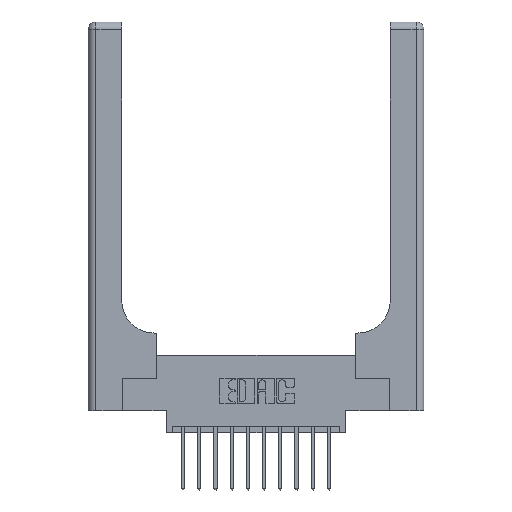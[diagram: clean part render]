
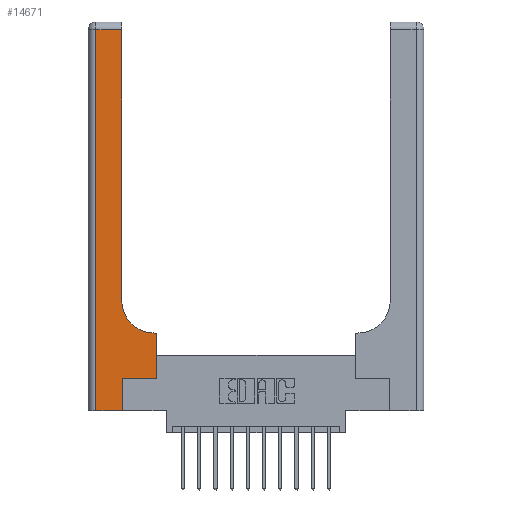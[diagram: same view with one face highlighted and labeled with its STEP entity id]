
A CAD part, top view. The second image highlights one B-rep face of the part: STEP entity #14671.
In plain terms, the highlighted planar face has unit normal (0, 0, 1).
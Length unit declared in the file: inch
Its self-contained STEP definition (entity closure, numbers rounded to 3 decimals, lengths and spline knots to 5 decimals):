
#357 = CARTESIAN_POINT ( 'NONE',  ( 0.51, 0.6, 0.37 ) ) ;
#471 = ORIENTED_EDGE ( 'NONE', *, *, #7750, .T. ) ;
#612 = VERTEX_POINT ( 'NONE', #16374 ) ;
#995 = CARTESIAN_POINT ( 'NONE',  ( 0., 2.94, 0.37 ) ) ;
#1033 = VERTEX_POINT ( 'NONE', #2273 ) ;
#1139 = CARTESIAN_POINT ( 'NONE',  ( 0.51, 0.85, 0.37 ) ) ;
#1230 = DIRECTION ( 'NONE',  ( 0., 1., 0. ) ) ;
#1379 = DIRECTION ( 'NONE',  ( 0., 0., -1. ) ) ;
#1489 = EDGE_CURVE ( 'NONE', #6824, #1033, #14939, .T. ) ;
#1620 = EDGE_CURVE ( 'NONE', #1694, #13149, #15596, .T. ) ;
#1694 = VERTEX_POINT ( 'NONE', #2983 ) ;
#1734 = DIRECTION ( 'NONE',  ( -1., 0., 0. ) ) ;
#1769 = ORIENTED_EDGE ( 'NONE', *, *, #6331, .T. ) ;
#1899 = VECTOR ( 'NONE', #1230, 39.37008 ) ;
#2103 = VERTEX_POINT ( 'NONE', #357 ) ;
#2273 = CARTESIAN_POINT ( 'NONE',  ( 0.528, 0.6, 0.37 ) ) ;
#2275 = LINE ( 'NONE', #995, #11332 ) ;
#2460 = ORIENTED_EDGE ( 'NONE', *, *, #1489, .T. ) ;
#2656 = DIRECTION ( 'NONE',  ( 1., 0., 0. ) ) ;
#2983 = CARTESIAN_POINT ( 'NONE',  ( 0.06, 0., 0.37 ) ) ;
#3029 = EDGE_CURVE ( 'NONE', #3965, #1694, #3734, .T. ) ;
#3409 = ORIENTED_EDGE ( 'NONE', *, *, #9407, .T. ) ;
#3491 = DIRECTION ( 'NONE',  ( 0., -1., 0. ) ) ;
#3734 = LINE ( 'NONE', #7376, #9521 ) ;
#3820 = VECTOR ( 'NONE', #11025, 39.37008 ) ;
#3836 = LINE ( 'NONE', #5083, #1899 ) ;
#3965 = VERTEX_POINT ( 'NONE', #11967 ) ;
#4679 = VECTOR ( 'NONE', #2656, 39.37008 ) ;
#4692 = DIRECTION ( 'NONE',  ( 0., 1., 0. ) ) ;
#4909 = VECTOR ( 'NONE', #15221, 39.37008 ) ;
#5016 = CARTESIAN_POINT ( 'NONE',  ( 0.528, 0.25, 0.37 ) ) ;
#5083 = CARTESIAN_POINT ( 'NONE',  ( 0.26, 3., 0.37 ) ) ;
#5941 = CIRCLE ( 'NONE', #9971, 0.25 ) ;
#6060 = CARTESIAN_POINT ( 'NONE',  ( 0.265, 0.25, 0.37 ) ) ;
#6062 = ORIENTED_EDGE ( 'NONE', *, *, #7723, .T. ) ;
#6219 = LINE ( 'NONE', #11360, #4909 ) ;
#6281 = VECTOR ( 'NONE', #14201, 39.37008 ) ;
#6331 = EDGE_CURVE ( 'NONE', #612, #3965, #2275, .T. ) ;
#6460 = AXIS2_PLACEMENT_3D ( 'NONE', #16609, #14115, #1734 ) ;
#6824 = VERTEX_POINT ( 'NONE', #15521 ) ;
#7288 = VERTEX_POINT ( 'NONE', #6060 ) ;
#7376 = CARTESIAN_POINT ( 'NONE',  ( 0.06, 3., 0.37 ) ) ;
#7723 = EDGE_CURVE ( 'NONE', #11399, #612, #3836, .T. ) ;
#7750 = EDGE_CURVE ( 'NONE', #2103, #11399, #5941, .T. ) ;
#7817 = PLANE ( 'NONE',  #6460 ) ;
#7854 = VECTOR ( 'NONE', #4692, 39.37008 ) ;
#8933 = ORIENTED_EDGE ( 'NONE', *, *, #3029, .T. ) ;
#8989 = CARTESIAN_POINT ( 'NONE',  ( 0., 0., 0.37 ) ) ;
#9015 = FACE_OUTER_BOUND ( 'NONE', #11273, .T. ) ;
#9031 = LINE ( 'NONE', #11518, #6281 ) ;
#9407 = EDGE_CURVE ( 'NONE', #13149, #7288, #13312, .T. ) ;
#9521 = VECTOR ( 'NONE', #3491, 39.37008 ) ;
#9588 = EDGE_CURVE ( 'NONE', #7288, #6824, #6219, .T. ) ;
#9788 = CARTESIAN_POINT ( 'NONE',  ( 0.265, 0., 0.37 ) ) ;
#9971 = AXIS2_PLACEMENT_3D ( 'NONE', #1139, #1379, #11649 ) ;
#10951 = EDGE_CURVE ( 'NONE', #1033, #2103, #9031, .T. ) ;
#11025 = DIRECTION ( 'NONE',  ( 0., 1., 0. ) ) ;
#11082 = CARTESIAN_POINT ( 'NONE',  ( 0.265, 0., 0.37 ) ) ;
#11088 = ORIENTED_EDGE ( 'NONE', *, *, #1620, .T. ) ;
#11227 = ORIENTED_EDGE ( 'NONE', *, *, #9588, .T. ) ;
#11273 = EDGE_LOOP ( 'NONE', ( #6062, #1769, #8933, #11088, #3409, #11227, #2460, #14259, #471 ) ) ;
#11332 = VECTOR ( 'NONE', #12771, 39.37008 ) ;
#11360 = CARTESIAN_POINT ( 'NONE',  ( 0.265, 0.25, 0.37 ) ) ;
#11399 = VERTEX_POINT ( 'NONE', #11815 ) ;
#11518 = CARTESIAN_POINT ( 'NONE',  ( 0.26, 0.6, 0.37 ) ) ;
#11649 = DIRECTION ( 'NONE',  ( 1., 0., 0. ) ) ;
#11815 = CARTESIAN_POINT ( 'NONE',  ( 0.26, 0.85, 0.37 ) ) ;
#11967 = CARTESIAN_POINT ( 'NONE',  ( 0.06, 2.94, 0.37 ) ) ;
#12771 = DIRECTION ( 'NONE',  ( -1., 0., 0. ) ) ;
#13149 = VERTEX_POINT ( 'NONE', #11082 ) ;
#13312 = LINE ( 'NONE', #9788, #3820 ) ;
#14115 = DIRECTION ( 'NONE',  ( 0., 0., -1. ) ) ;
#14201 = DIRECTION ( 'NONE',  ( -1., 0., 0. ) ) ;
#14259 = ORIENTED_EDGE ( 'NONE', *, *, #10951, .T. ) ;
#14671 = ADVANCED_FACE ( 'NONE', ( #9015 ), #7817, .F. ) ;
#14939 = LINE ( 'NONE', #5016, #7854 ) ;
#15221 = DIRECTION ( 'NONE',  ( 1., 0., 0. ) ) ;
#15521 = CARTESIAN_POINT ( 'NONE',  ( 0.528, 0.25, 0.37 ) ) ;
#15596 = LINE ( 'NONE', #8989, #4679 ) ;
#16374 = CARTESIAN_POINT ( 'NONE',  ( 0.26, 2.94, 0.37 ) ) ;
#16609 = CARTESIAN_POINT ( 'NONE',  ( 0., 3., 0.37 ) ) ;
